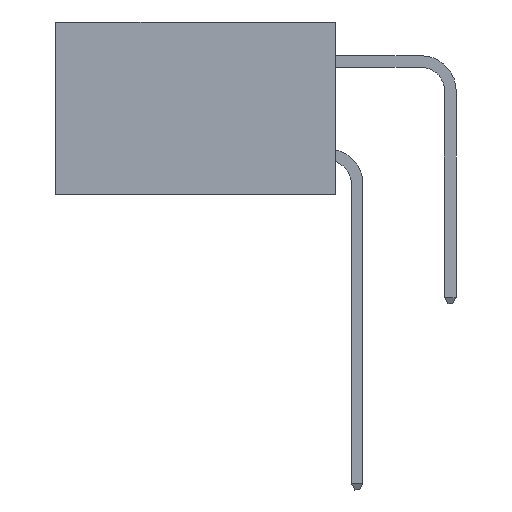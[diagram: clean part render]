
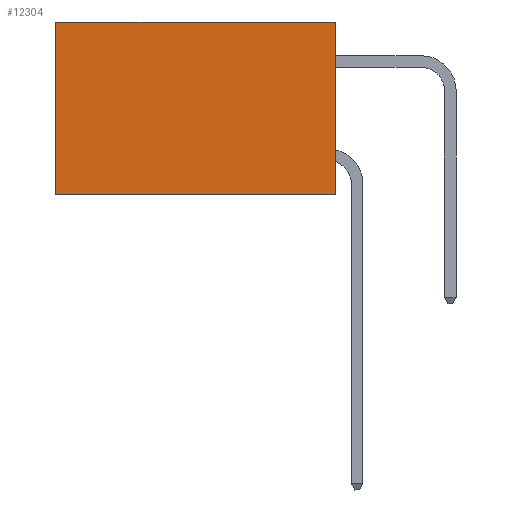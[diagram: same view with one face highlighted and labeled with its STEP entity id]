
A CAD part, left-side view. The second image highlights one B-rep face of the part: STEP entity #12304.
In plain terms, the highlighted planar face has unit normal (-1, 0, 0).
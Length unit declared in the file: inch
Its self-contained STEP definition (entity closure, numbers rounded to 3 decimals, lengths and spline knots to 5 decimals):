
#85 = EDGE_CURVE ( 'NONE', #22016, #10669, #13415, .T. ) ;
#846 = VECTOR ( 'NONE', #2523, 39.37008 ) ;
#1168 = LINE ( 'NONE', #12019, #14092 ) ;
#1479 = AXIS2_PLACEMENT_3D ( 'NONE', #20848, #27798, #18732 ) ;
#2523 = DIRECTION ( 'NONE',  ( 0., 0., -1. ) ) ;
#3930 = LINE ( 'NONE', #24247, #5003 ) ;
#5003 = VECTOR ( 'NONE', #8052, 39.37008 ) ;
#7422 = VERTEX_POINT ( 'NONE', #8262 ) ;
#8052 = DIRECTION ( 'NONE',  ( 0., 0., -1. ) ) ;
#8262 = CARTESIAN_POINT ( 'NONE',  ( 0.2875, 0.6, -0.37 ) ) ;
#8900 = FACE_OUTER_BOUND ( 'NONE', #13905, .T. ) ;
#9202 = ORIENTED_EDGE ( 'NONE', *, *, #85, .T. ) ;
#10669 = VERTEX_POINT ( 'NONE', #24180 ) ;
#12019 = CARTESIAN_POINT ( 'NONE',  ( 0.2875, 0., -0.37 ) ) ;
#12095 = ORIENTED_EDGE ( 'NONE', *, *, #15128, .F. ) ;
#12304 = ADVANCED_FACE ( 'NONE', ( #8900 ), #28093, .F. ) ;
#12414 = VERTEX_POINT ( 'NONE', #26178 ) ;
#13372 = LINE ( 'NONE', #25641, #846 ) ;
#13415 = LINE ( 'NONE', #24212, #25338 ) ;
#13905 = EDGE_LOOP ( 'NONE', ( #14209, #27233, #12095, #9202 ) ) ;
#14092 = VECTOR ( 'NONE', #28474, 39.37008 ) ;
#14209 = ORIENTED_EDGE ( 'NONE', *, *, #27800, .T. ) ;
#15045 = DIRECTION ( 'NONE',  ( 0., 1., 0. ) ) ;
#15128 = EDGE_CURVE ( 'NONE', #22016, #12414, #13372, .T. ) ;
#18732 = DIRECTION ( 'NONE',  ( 0., 0., -1. ) ) ;
#20848 = CARTESIAN_POINT ( 'NONE',  ( 0.2875, 0., 0. ) ) ;
#21599 = CARTESIAN_POINT ( 'NONE',  ( 0.2875, 0., 0. ) ) ;
#22016 = VERTEX_POINT ( 'NONE', #21599 ) ;
#24180 = CARTESIAN_POINT ( 'NONE',  ( 0.2875, 0.6, 0. ) ) ;
#24212 = CARTESIAN_POINT ( 'NONE',  ( 0.2875, 0., 0. ) ) ;
#24247 = CARTESIAN_POINT ( 'NONE',  ( 0.2875, 0.6, 0. ) ) ;
#25338 = VECTOR ( 'NONE', #15045, 39.37008 ) ;
#25641 = CARTESIAN_POINT ( 'NONE',  ( 0.2875, 0., 0. ) ) ;
#25673 = EDGE_CURVE ( 'NONE', #12414, #7422, #1168, .T. ) ;
#26178 = CARTESIAN_POINT ( 'NONE',  ( 0.2875, 0., -0.37 ) ) ;
#27233 = ORIENTED_EDGE ( 'NONE', *, *, #25673, .F. ) ;
#27798 = DIRECTION ( 'NONE',  ( 1., 0., 0. ) ) ;
#27800 = EDGE_CURVE ( 'NONE', #10669, #7422, #3930, .T. ) ;
#28093 = PLANE ( 'NONE',  #1479 ) ;
#28474 = DIRECTION ( 'NONE',  ( 0., 1., 0. ) ) ;
